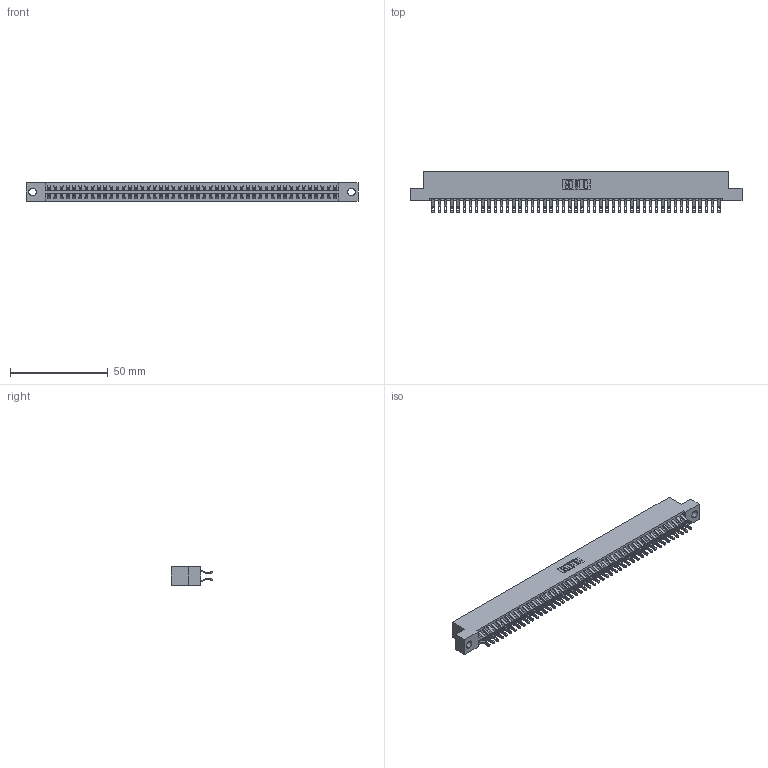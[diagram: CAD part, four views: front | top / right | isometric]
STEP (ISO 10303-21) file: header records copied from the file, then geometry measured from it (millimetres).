
FILE_DESCRIPTION (( 'STEP AP203' ), '1' );
FILE_NAME ('346-094-555-204.STEP', '2022-05-26T14:51:38', ( '' ), ( '' ), 'SwSTEP 2.0', 'SolidWorks 2020', '' );
FILE_SCHEMA (( 'CONFIG_CONTROL_DESIGN' ));
Length unit declared in the file: inch
Products named in the file (3): 345-292-001_555 Tail; 346-094-555-204; 346 Part_Flush Mounting Lugs - 0.156 Dia-TH
Assembly tree (95 placements, depth 2):
  346-094-555-204
    346 Part_Flush Mounting Lugs - 0.156 Dia-TH
    345-292-001_555 Tail  x94
Bounding box: 169.8 x 21.46 x 9.4 mm (x, y, z)
Volume: 16763 mm3; surface area: 23940.3 mm2
Topology: 95 solids, 95 shells, 5588 faces, 17567 edges, 11710 vertices
Faces by surface type: plane 3192, cylinder 2396
Entity records: 30745 total; most frequent: CARTESIAN_POINT 5100, ORIENTED_EDGE 5002, DIRECTION 4513, EDGE_CURVE 2501, LINE 2161, VECTOR 2161, VERTEX_POINT 1666, AXIS2_PLACEMENT_3D 1176
